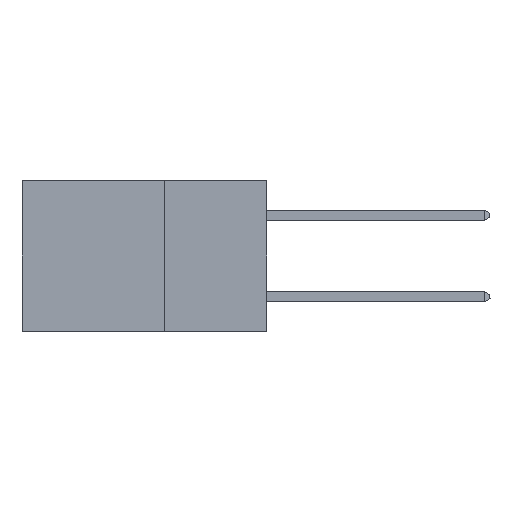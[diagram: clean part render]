
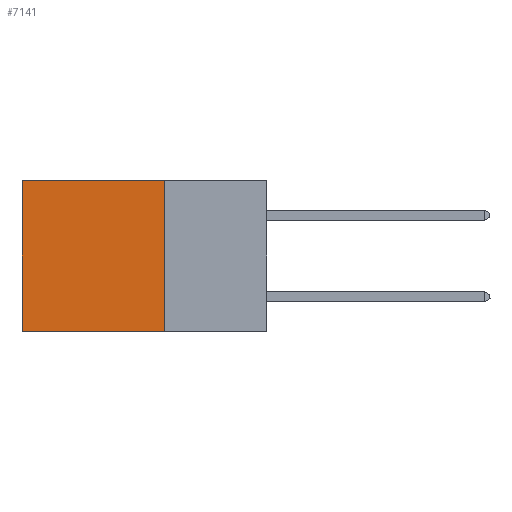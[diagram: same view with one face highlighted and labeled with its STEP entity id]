
A CAD part, left-side view. The second image highlights one B-rep face of the part: STEP entity #7141.
In plain terms, the highlighted planar face has unit normal (-1, 0, 0).
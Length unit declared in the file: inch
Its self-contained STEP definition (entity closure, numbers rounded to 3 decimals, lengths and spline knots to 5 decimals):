
#614 = EDGE_CURVE ( 'NONE', #15147, #4981, #6605, .T. ) ;
#627 = FACE_OUTER_BOUND ( 'NONE', #8937, .T. ) ;
#753 = ORIENTED_EDGE ( 'NONE', *, *, #2736, .F. ) ;
#1035 = DIRECTION ( 'NONE',  ( 0., 0., -1. ) ) ;
#1663 = PLANE ( 'NONE',  #11718 ) ;
#1754 = CARTESIAN_POINT ( 'NONE',  ( 0.2875, 0.25, 0. ) ) ;
#2246 = CARTESIAN_POINT ( 'NONE',  ( 0.2875, 0.6, 0. ) ) ;
#2266 = DIRECTION ( 'NONE',  ( 0., 0., -1. ) ) ;
#2675 = CARTESIAN_POINT ( 'NONE',  ( 0.2875, 0.25, 0. ) ) ;
#2736 = EDGE_CURVE ( 'NONE', #5817, #10998, #14441, .T. ) ;
#2800 = ORIENTED_EDGE ( 'NONE', *, *, #614, .T. ) ;
#2930 = ORIENTED_EDGE ( 'NONE', *, *, #6816, .T. ) ;
#3706 = ORIENTED_EDGE ( 'NONE', *, *, #11057, .F. ) ;
#4981 = VERTEX_POINT ( 'NONE', #14690 ) ;
#5528 = VECTOR ( 'NONE', #2266, 39.37008 ) ;
#5817 = VERTEX_POINT ( 'NONE', #14566 ) ;
#6573 = DIRECTION ( 'NONE',  ( 0., 0., -1. ) ) ;
#6605 = LINE ( 'NONE', #2675, #11763 ) ;
#6816 = EDGE_CURVE ( 'NONE', #4981, #10998, #13328, .T. ) ;
#7141 = ADVANCED_FACE ( 'NONE', ( #627 ), #1663, .F. ) ;
#7380 = CARTESIAN_POINT ( 'NONE',  ( 0.2875, 0.25, -0.37 ) ) ;
#8937 = EDGE_LOOP ( 'NONE', ( #2930, #753, #3706, #2800 ) ) ;
#9653 = DIRECTION ( 'NONE',  ( 0., 1., 0. ) ) ;
#9915 = VECTOR ( 'NONE', #1035, 39.37008 ) ;
#10317 = DIRECTION ( 'NONE',  ( 0., 1., 0. ) ) ;
#10403 = CARTESIAN_POINT ( 'NONE',  ( 0.2875, 0.6, -0.37 ) ) ;
#10998 = VERTEX_POINT ( 'NONE', #10403 ) ;
#11029 = VECTOR ( 'NONE', #9653, 39.37008 ) ;
#11057 = EDGE_CURVE ( 'NONE', #15147, #5817, #11922, .T. ) ;
#11718 = AXIS2_PLACEMENT_3D ( 'NONE', #1754, #13002, #6573 ) ;
#11763 = VECTOR ( 'NONE', #10317, 39.37008 ) ;
#11922 = LINE ( 'NONE', #15593, #5528 ) ;
#13002 = DIRECTION ( 'NONE',  ( 1., 0., 0. ) ) ;
#13328 = LINE ( 'NONE', #2246, #9915 ) ;
#14236 = CARTESIAN_POINT ( 'NONE',  ( 0.2875, 0.25, 0. ) ) ;
#14441 = LINE ( 'NONE', #7380, #11029 ) ;
#14566 = CARTESIAN_POINT ( 'NONE',  ( 0.2875, 0.25, -0.37 ) ) ;
#14690 = CARTESIAN_POINT ( 'NONE',  ( 0.2875, 0.6, 0. ) ) ;
#15147 = VERTEX_POINT ( 'NONE', #14236 ) ;
#15593 = CARTESIAN_POINT ( 'NONE',  ( 0.2875, 0.25, 0. ) ) ;
